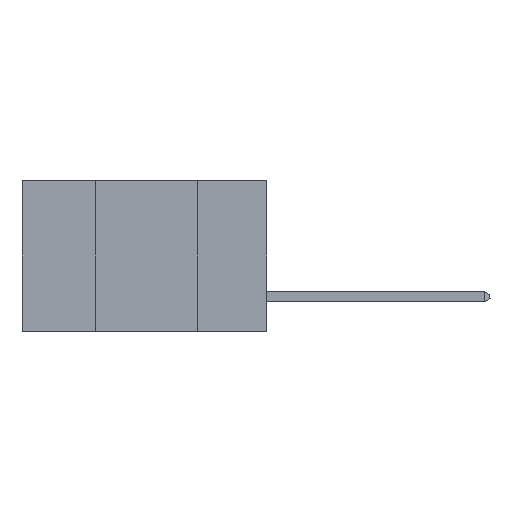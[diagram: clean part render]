
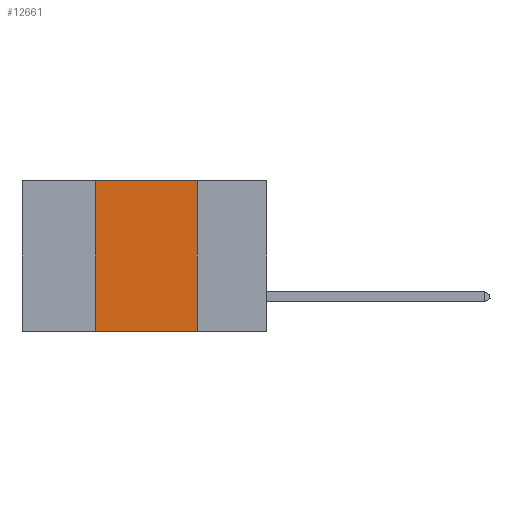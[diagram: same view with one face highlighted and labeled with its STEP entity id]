
A CAD part, left-side view. The second image highlights one B-rep face of the part: STEP entity #12661.
In plain terms, the highlighted planar face has unit normal (-1, 0, 0).
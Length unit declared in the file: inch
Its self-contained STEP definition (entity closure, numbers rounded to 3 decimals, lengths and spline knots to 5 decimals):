
#2009 = VECTOR ( 'NONE', #16059, 39.37008 ) ;
#2020 = EDGE_LOOP ( 'NONE', ( #4278, #18753, #13197, #17365 ) ) ;
#2346 = CARTESIAN_POINT ( 'NONE',  ( 0., 0.17, 0. ) ) ;
#2914 = LINE ( 'NONE', #11596, #4141 ) ;
#3161 = CARTESIAN_POINT ( 'NONE',  ( 0., 0.6, -0.37 ) ) ;
#4141 = VECTOR ( 'NONE', #18207, 39.37008 ) ;
#4278 = ORIENTED_EDGE ( 'NONE', *, *, #8235, .F. ) ;
#5617 = VECTOR ( 'NONE', #11393, 39.37008 ) ;
#6205 = LINE ( 'NONE', #3161, #2009 ) ;
#7123 = EDGE_CURVE ( 'NONE', #9391, #16455, #18626, .T. ) ;
#7739 = DIRECTION ( 'NONE',  ( 1., 0., 0. ) ) ;
#7824 = LINE ( 'NONE', #17868, #5617 ) ;
#8097 = CARTESIAN_POINT ( 'NONE',  ( 0., 0.42, 0. ) ) ;
#8235 = EDGE_CURVE ( 'NONE', #12012, #10583, #7824, .T. ) ;
#9391 = VERTEX_POINT ( 'NONE', #11844 ) ;
#9633 = AXIS2_PLACEMENT_3D ( 'NONE', #15490, #7739, #17200 ) ;
#10583 = VERTEX_POINT ( 'NONE', #11057 ) ;
#11057 = CARTESIAN_POINT ( 'NONE',  ( 0., 0.17, -0.37 ) ) ;
#11393 = DIRECTION ( 'NONE',  ( 0., 0., -1. ) ) ;
#11596 = CARTESIAN_POINT ( 'NONE',  ( 0., 0.6, 0. ) ) ;
#11844 = CARTESIAN_POINT ( 'NONE',  ( 0., 0.42, -0.37 ) ) ;
#12012 = VERTEX_POINT ( 'NONE', #2346 ) ;
#12580 = VECTOR ( 'NONE', #17258, 39.37008 ) ;
#12661 = ADVANCED_FACE ( 'NONE', ( #13735 ), #18721, .F. ) ;
#13197 = ORIENTED_EDGE ( 'NONE', *, *, #7123, .F. ) ;
#13735 = FACE_OUTER_BOUND ( 'NONE', #2020, .T. ) ;
#15490 = CARTESIAN_POINT ( 'NONE',  ( 0., 0.6, 0. ) ) ;
#15627 = CARTESIAN_POINT ( 'NONE',  ( 0., 0.42, 0. ) ) ;
#15696 = EDGE_CURVE ( 'NONE', #16455, #12012, #2914, .T. ) ;
#16059 = DIRECTION ( 'NONE',  ( 0., -1., 0. ) ) ;
#16455 = VERTEX_POINT ( 'NONE', #8097 ) ;
#17200 = DIRECTION ( 'NONE',  ( 0., 0., -1. ) ) ;
#17258 = DIRECTION ( 'NONE',  ( 0., 0., 1. ) ) ;
#17365 = ORIENTED_EDGE ( 'NONE', *, *, #18752, .T. ) ;
#17868 = CARTESIAN_POINT ( 'NONE',  ( 0., 0.17, 0. ) ) ;
#18207 = DIRECTION ( 'NONE',  ( 0., -1., 0. ) ) ;
#18626 = LINE ( 'NONE', #15627, #12580 ) ;
#18721 = PLANE ( 'NONE',  #9633 ) ;
#18752 = EDGE_CURVE ( 'NONE', #9391, #10583, #6205, .T. ) ;
#18753 = ORIENTED_EDGE ( 'NONE', *, *, #15696, .F. ) ;
